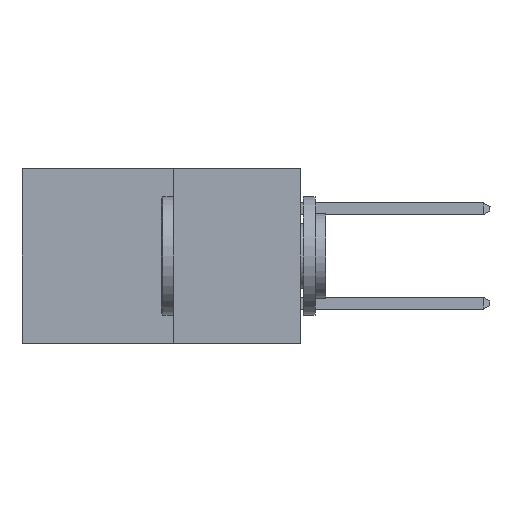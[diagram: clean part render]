
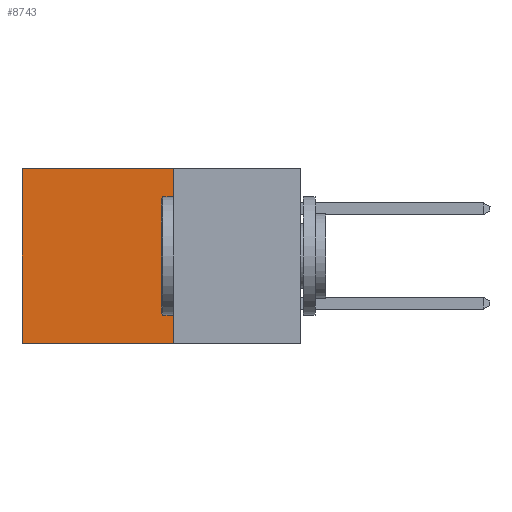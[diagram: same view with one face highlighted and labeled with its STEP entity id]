
A CAD part, left-side view. The second image highlights one B-rep face of the part: STEP entity #8743.
In plain terms, the highlighted planar face has unit normal (-1, 0, 0).
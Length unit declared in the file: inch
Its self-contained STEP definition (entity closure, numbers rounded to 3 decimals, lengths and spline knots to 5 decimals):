
#137 = EDGE_CURVE ( 'NONE', #7899, #7316, #7677, .T. ) ;
#1672 = DIRECTION ( 'NONE',  ( 1., 0., 0. ) ) ;
#2663 = FACE_OUTER_BOUND ( 'NONE', #3721, .T. ) ;
#2830 = DIRECTION ( 'NONE',  ( 0., 1., 0. ) ) ;
#3028 = VECTOR ( 'NONE', #2830, 39.37008 ) ;
#3505 = VECTOR ( 'NONE', #7425, 39.37008 ) ;
#3721 = EDGE_LOOP ( 'NONE', ( #4226, #4325, #4333, #4419 ) ) ;
#3796 = LINE ( 'NONE', #7493, #3505 ) ;
#3859 = VECTOR ( 'NONE', #7578, 39.37008 ) ;
#4226 = ORIENTED_EDGE ( 'NONE', *, *, #6164, .T. ) ;
#4325 = ORIENTED_EDGE ( 'NONE', *, *, #6127, .F. ) ;
#4333 = ORIENTED_EDGE ( 'NONE', *, *, #137, .F. ) ;
#4419 = ORIENTED_EDGE ( 'NONE', *, *, #4737, .T. ) ;
#4587 = CARTESIAN_POINT ( 'NONE',  ( 0.277, 0.59, 0. ) ) ;
#4617 = LINE ( 'NONE', #8997, #11112 ) ;
#4686 = CARTESIAN_POINT ( 'NONE',  ( 0.277, 0.27, 0. ) ) ;
#4737 = EDGE_CURVE ( 'NONE', #7899, #6063, #3796, .T. ) ;
#5852 = CARTESIAN_POINT ( 'NONE',  ( 0.277, 0.27, -0.37 ) ) ;
#6063 = VERTEX_POINT ( 'NONE', #4587 ) ;
#6127 = EDGE_CURVE ( 'NONE', #7316, #7709, #7187, .T. ) ;
#6164 = EDGE_CURVE ( 'NONE', #6063, #7709, #4617, .T. ) ;
#6319 = CARTESIAN_POINT ( 'NONE',  ( 0.277, 0.27, -0.37 ) ) ;
#7187 = LINE ( 'NONE', #8963, #3028 ) ;
#7197 = PLANE ( 'NONE',  #10042 ) ;
#7210 = CARTESIAN_POINT ( 'NONE',  ( 0.277, 0.27, -0.37 ) ) ;
#7316 = VERTEX_POINT ( 'NONE', #5852 ) ;
#7425 = DIRECTION ( 'NONE',  ( 0., 1., 0. ) ) ;
#7493 = CARTESIAN_POINT ( 'NONE',  ( 0.277, 0.27, 0. ) ) ;
#7578 = DIRECTION ( 'NONE',  ( 0., 0., -1. ) ) ;
#7677 = LINE ( 'NONE', #7210, #3859 ) ;
#7709 = VERTEX_POINT ( 'NONE', #7959 ) ;
#7899 = VERTEX_POINT ( 'NONE', #4686 ) ;
#7959 = CARTESIAN_POINT ( 'NONE',  ( 0.277, 0.59, -0.37 ) ) ;
#8060 = DIRECTION ( 'NONE',  ( 0., 0., -1. ) ) ;
#8743 = ADVANCED_FACE ( 'NONE', ( #2663 ), #7197, .F. ) ;
#8963 = CARTESIAN_POINT ( 'NONE',  ( 0.277, 0.27, -0.37 ) ) ;
#8997 = CARTESIAN_POINT ( 'NONE',  ( 0.277, 0.59, -0.37 ) ) ;
#9851 = DIRECTION ( 'NONE',  ( 0., 0., -1. ) ) ;
#10042 = AXIS2_PLACEMENT_3D ( 'NONE', #6319, #1672, #8060 ) ;
#11112 = VECTOR ( 'NONE', #9851, 39.37008 ) ;
